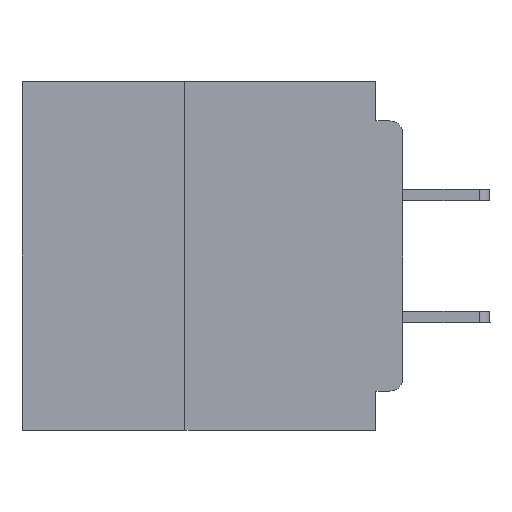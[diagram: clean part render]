
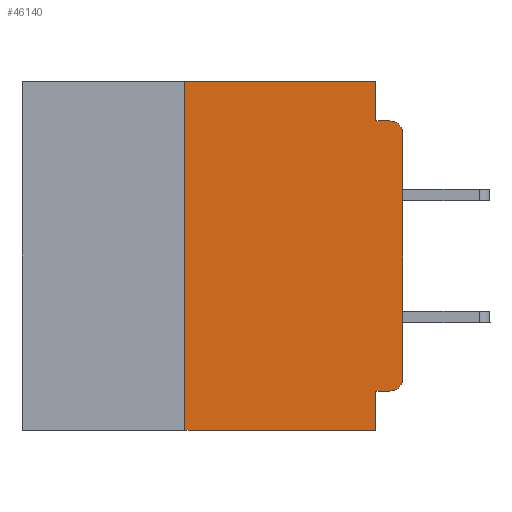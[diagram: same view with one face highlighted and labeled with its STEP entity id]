
A CAD part, left-side view. The second image highlights one B-rep face of the part: STEP entity #46140.
In plain terms, the highlighted planar face has unit normal (-1, 0, 0).
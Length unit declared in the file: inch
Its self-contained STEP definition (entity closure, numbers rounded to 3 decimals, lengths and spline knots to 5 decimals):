
#1030 = DIRECTION ( 'NONE',  ( 0., 0., -1. ) ) ;
#2585 = VERTEX_POINT ( 'NONE', #41561 ) ;
#2875 = AXIS2_PLACEMENT_3D ( 'NONE', #23941, #46944, #33309 ) ;
#3217 = LINE ( 'NONE', #27139, #17100 ) ;
#3651 = EDGE_LOOP ( 'NONE', ( #40873, #45181, #34397, #11106, #27873, #17004, #56632, #45919, #14818, #51621 ) ) ;
#4106 = CARTESIAN_POINT ( 'NONE',  ( 0., 0., -0.34 ) ) ;
#6035 = VERTEX_POINT ( 'NONE', #4106 ) ;
#6186 = CARTESIAN_POINT ( 'NONE',  ( 0., 0.015, -0.34 ) ) ;
#7396 = VERTEX_POINT ( 'NONE', #20043 ) ;
#8790 = LINE ( 'NONE', #9486, #56491 ) ;
#9375 = DIRECTION ( 'NONE',  ( 0., -1., 0. ) ) ;
#9486 = CARTESIAN_POINT ( 'NONE',  ( 0., 0., -0.355 ) ) ;
#9640 = VERTEX_POINT ( 'NONE', #54219 ) ;
#10843 = DIRECTION ( 'NONE',  ( 0., 0., -1. ) ) ;
#11106 = ORIENTED_EDGE ( 'NONE', *, *, #58591, .F. ) ;
#12431 = CARTESIAN_POINT ( 'NONE',  ( 0., 0.031, -0.4 ) ) ;
#13380 = VERTEX_POINT ( 'NONE', #40683 ) ;
#14164 = LINE ( 'NONE', #40658, #27999 ) ;
#14517 = FACE_OUTER_BOUND ( 'NONE', #3651, .T. ) ;
#14818 = ORIENTED_EDGE ( 'NONE', *, *, #20857, .F. ) ;
#15112 = LINE ( 'NONE', #46243, #38331 ) ;
#15417 = VERTEX_POINT ( 'NONE', #17096 ) ;
#17004 = ORIENTED_EDGE ( 'NONE', *, *, #55534, .F. ) ;
#17008 = LINE ( 'NONE', #21234, #40192 ) ;
#17096 = CARTESIAN_POINT ( 'NONE',  ( 0., 0.25, 0. ) ) ;
#17100 = VECTOR ( 'NONE', #54680, 39.37008 ) ;
#18121 = CIRCLE ( 'NONE', #48283, 0.015 ) ;
#20043 = CARTESIAN_POINT ( 'NONE',  ( 0., 0.031, -0.4 ) ) ;
#20857 = EDGE_CURVE ( 'NONE', #40233, #2585, #8790, .T. ) ;
#21234 = CARTESIAN_POINT ( 'NONE',  ( 0., 0.031, 0. ) ) ;
#21901 = CARTESIAN_POINT ( 'NONE',  ( 0., 0., -0.06 ) ) ;
#23941 = CARTESIAN_POINT ( 'NONE',  ( 0., 0.437, 0. ) ) ;
#24573 = VECTOR ( 'NONE', #36982, 39.37008 ) ;
#25367 = DIRECTION ( 'NONE',  ( 0., -1., 0. ) ) ;
#25948 = EDGE_CURVE ( 'NONE', #6035, #34898, #3217, .T. ) ;
#26132 = VECTOR ( 'NONE', #25367, 39.37008 ) ;
#27139 = CARTESIAN_POINT ( 'NONE',  ( 0., 0., 0. ) ) ;
#27873 = ORIENTED_EDGE ( 'NONE', *, *, #47162, .F. ) ;
#27999 = VECTOR ( 'NONE', #45258, 39.37008 ) ;
#28620 = PLANE ( 'NONE',  #2875 ) ;
#28909 = DIRECTION ( 'NONE',  ( -1., 0., 0. ) ) ;
#30670 = AXIS2_PLACEMENT_3D ( 'NONE', #56402, #28909, #1030 ) ;
#31145 = DIRECTION ( 'NONE',  ( 0., 0., -1. ) ) ;
#33309 = DIRECTION ( 'NONE',  ( 0., 0., -1. ) ) ;
#34397 = ORIENTED_EDGE ( 'NONE', *, *, #48697, .F. ) ;
#34850 = DIRECTION ( 'NONE',  ( 0., 0., -1. ) ) ;
#34898 = VERTEX_POINT ( 'NONE', #21901 ) ;
#35974 = VECTOR ( 'NONE', #31145, 39.37008 ) ;
#36982 = DIRECTION ( 'NONE',  ( 0., 0., 1. ) ) ;
#37387 = LINE ( 'NONE', #12431, #35974 ) ;
#38331 = VECTOR ( 'NONE', #9375, 39.37008 ) ;
#38353 = LINE ( 'NONE', #59789, #24573 ) ;
#38693 = DIRECTION ( 'NONE',  ( -1., 0., 0. ) ) ;
#40192 = VECTOR ( 'NONE', #34850, 39.37008 ) ;
#40210 = EDGE_CURVE ( 'NONE', #2585, #7396, #37387, .T. ) ;
#40233 = VERTEX_POINT ( 'NONE', #45032 ) ;
#40658 = CARTESIAN_POINT ( 'NONE',  ( 0., 0., -0.045 ) ) ;
#40683 = CARTESIAN_POINT ( 'NONE',  ( 0., 0.031, -0.045 ) ) ;
#40873 = ORIENTED_EDGE ( 'NONE', *, *, #25948, .T. ) ;
#41561 = CARTESIAN_POINT ( 'NONE',  ( 0., 0.031, -0.355 ) ) ;
#45032 = CARTESIAN_POINT ( 'NONE',  ( 0., 0.015, -0.355 ) ) ;
#45181 = ORIENTED_EDGE ( 'NONE', *, *, #59045, .T. ) ;
#45258 = DIRECTION ( 'NONE',  ( 0., -1., 0. ) ) ;
#45351 = VERTEX_POINT ( 'NONE', #48771 ) ;
#45919 = ORIENTED_EDGE ( 'NONE', *, *, #40210, .F. ) ;
#46140 = ADVANCED_FACE ( 'NONE', ( #14517 ), #28620, .F. ) ;
#46243 = CARTESIAN_POINT ( 'NONE',  ( 0., 0.437, 0. ) ) ;
#46336 = EDGE_CURVE ( 'NONE', #45351, #7396, #50594, .T. ) ;
#46770 = EDGE_CURVE ( 'NONE', #40233, #6035, #18121, .T. ) ;
#46944 = DIRECTION ( 'NONE',  ( 1., 0., 0. ) ) ;
#47162 = EDGE_CURVE ( 'NONE', #15417, #9640, #15112, .T. ) ;
#48283 = AXIS2_PLACEMENT_3D ( 'NONE', #6186, #38693, #10843 ) ;
#48333 = CARTESIAN_POINT ( 'NONE',  ( 0., 0.437, -0.4 ) ) ;
#48697 = EDGE_CURVE ( 'NONE', #13380, #55804, #14164, .T. ) ;
#48771 = CARTESIAN_POINT ( 'NONE',  ( 0., 0.25, -0.4 ) ) ;
#50594 = LINE ( 'NONE', #48333, #26132 ) ;
#51134 = DIRECTION ( 'NONE',  ( 0., 1., 0. ) ) ;
#51621 = ORIENTED_EDGE ( 'NONE', *, *, #46770, .T. ) ;
#52246 = CIRCLE ( 'NONE', #30670, 0.015 ) ;
#52519 = CARTESIAN_POINT ( 'NONE',  ( 0., 0.015, -0.045 ) ) ;
#54219 = CARTESIAN_POINT ( 'NONE',  ( 0., 0.031, 0. ) ) ;
#54680 = DIRECTION ( 'NONE',  ( 0., 0., 1. ) ) ;
#55534 = EDGE_CURVE ( 'NONE', #45351, #15417, #38353, .T. ) ;
#55804 = VERTEX_POINT ( 'NONE', #52519 ) ;
#56402 = CARTESIAN_POINT ( 'NONE',  ( 0., 0.015, -0.06 ) ) ;
#56491 = VECTOR ( 'NONE', #51134, 39.37008 ) ;
#56632 = ORIENTED_EDGE ( 'NONE', *, *, #46336, .T. ) ;
#58591 = EDGE_CURVE ( 'NONE', #9640, #13380, #17008, .T. ) ;
#59045 = EDGE_CURVE ( 'NONE', #34898, #55804, #52246, .T. ) ;
#59789 = CARTESIAN_POINT ( 'NONE',  ( 0., 0.25, -0.4 ) ) ;
